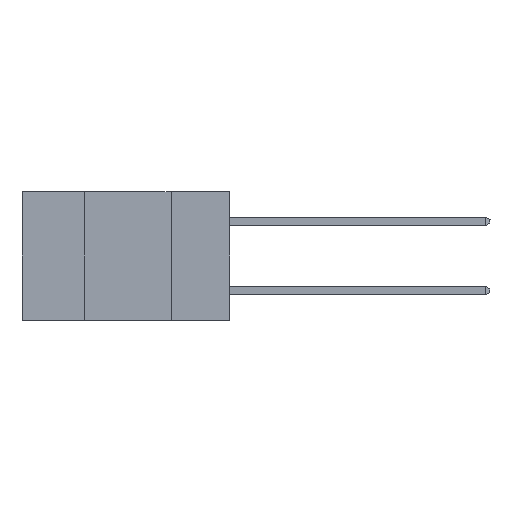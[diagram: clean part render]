
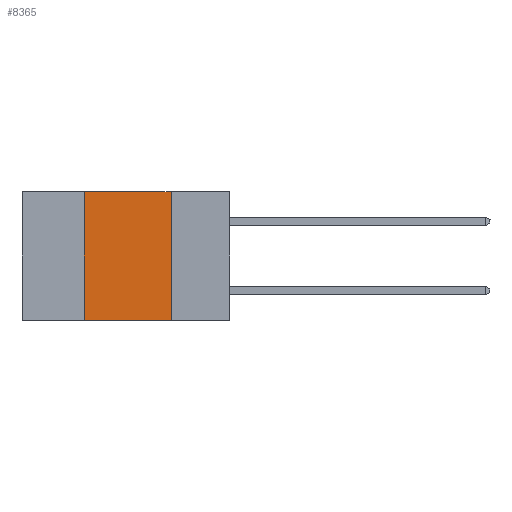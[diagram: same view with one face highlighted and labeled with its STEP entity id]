
A CAD part, left-side view. The second image highlights one B-rep face of the part: STEP entity #8365.
In plain terms, the highlighted planar face has unit normal (-1, 0, 0).
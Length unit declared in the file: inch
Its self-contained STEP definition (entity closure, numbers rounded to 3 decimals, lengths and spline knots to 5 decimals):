
#151 = CARTESIAN_POINT ( 'NONE',  ( 0., 0.42, 0. ) ) ;
#520 = DIRECTION ( 'NONE',  ( 1., 0., 0. ) ) ;
#719 = EDGE_CURVE ( 'NONE', #3000, #6849, #6869, .T. ) ;
#833 = ORIENTED_EDGE ( 'NONE', *, *, #2470, .F. ) ;
#1400 = VECTOR ( 'NONE', #10133, 39.37008 ) ;
#1420 = ORIENTED_EDGE ( 'NONE', *, *, #4231, .F. ) ;
#1459 = CARTESIAN_POINT ( 'NONE',  ( 0., 0.17, 0. ) ) ;
#2314 = EDGE_LOOP ( 'NONE', ( #833, #5556, #1420, #8359 ) ) ;
#2470 = EDGE_CURVE ( 'NONE', #3389, #6849, #7210, .T. ) ;
#2624 = VERTEX_POINT ( 'NONE', #151 ) ;
#2642 = CARTESIAN_POINT ( 'NONE',  ( 0., 0.6, 0. ) ) ;
#3000 = VERTEX_POINT ( 'NONE', #10118 ) ;
#3389 = VERTEX_POINT ( 'NONE', #7056 ) ;
#3663 = LINE ( 'NONE', #2642, #8901 ) ;
#3771 = CARTESIAN_POINT ( 'NONE',  ( 0., 0.42, 0. ) ) ;
#3840 = DIRECTION ( 'NONE',  ( 0., -1., 0. ) ) ;
#4104 = DIRECTION ( 'NONE',  ( 0., 0., -1. ) ) ;
#4156 = EDGE_CURVE ( 'NONE', #2624, #3389, #3663, .T. ) ;
#4231 = EDGE_CURVE ( 'NONE', #3000, #2624, #6734, .T. ) ;
#4258 = VECTOR ( 'NONE', #11214, 39.37008 ) ;
#5468 = DIRECTION ( 'NONE',  ( 0., -1., 0. ) ) ;
#5556 = ORIENTED_EDGE ( 'NONE', *, *, #4156, .F. ) ;
#5798 = AXIS2_PLACEMENT_3D ( 'NONE', #8844, #520, #4104 ) ;
#6734 = LINE ( 'NONE', #3771, #4258 ) ;
#6849 = VERTEX_POINT ( 'NONE', #8232 ) ;
#6869 = LINE ( 'NONE', #7525, #10563 ) ;
#7056 = CARTESIAN_POINT ( 'NONE',  ( 0., 0.17, 0. ) ) ;
#7210 = LINE ( 'NONE', #1459, #1400 ) ;
#7364 = FACE_OUTER_BOUND ( 'NONE', #2314, .T. ) ;
#7525 = CARTESIAN_POINT ( 'NONE',  ( 0., 0.6, -0.37 ) ) ;
#7867 = PLANE ( 'NONE',  #5798 ) ;
#8232 = CARTESIAN_POINT ( 'NONE',  ( 0., 0.17, -0.37 ) ) ;
#8359 = ORIENTED_EDGE ( 'NONE', *, *, #719, .T. ) ;
#8365 = ADVANCED_FACE ( 'NONE', ( #7364 ), #7867, .F. ) ;
#8844 = CARTESIAN_POINT ( 'NONE',  ( 0., 0.6, 0. ) ) ;
#8901 = VECTOR ( 'NONE', #5468, 39.37008 ) ;
#10118 = CARTESIAN_POINT ( 'NONE',  ( 0., 0.42, -0.37 ) ) ;
#10133 = DIRECTION ( 'NONE',  ( 0., 0., -1. ) ) ;
#10563 = VECTOR ( 'NONE', #3840, 39.37008 ) ;
#11214 = DIRECTION ( 'NONE',  ( 0., 0., 1. ) ) ;
